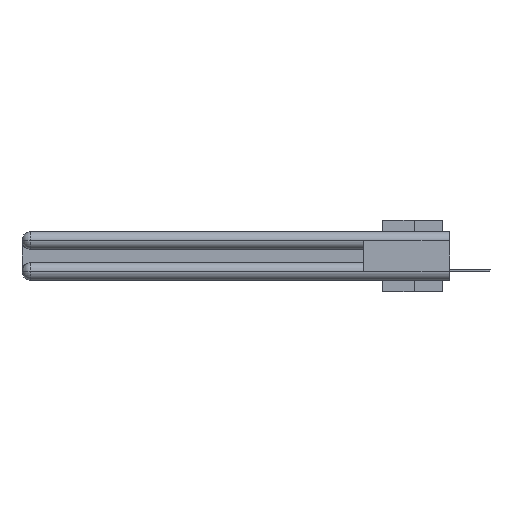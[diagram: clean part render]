
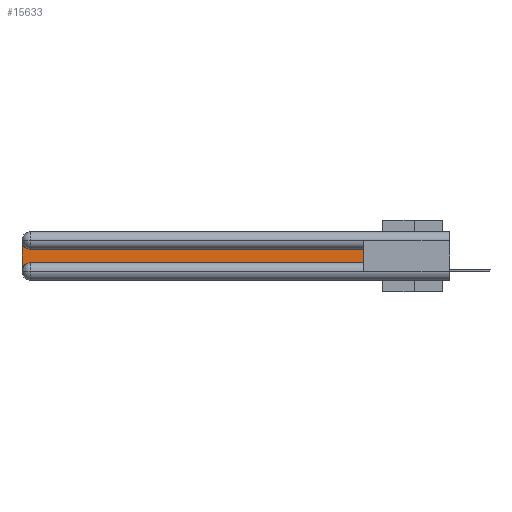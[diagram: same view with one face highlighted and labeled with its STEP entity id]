
A CAD part, left-side view. The second image highlights one B-rep face of the part: STEP entity #15633.
In plain terms, the highlighted planar face has unit normal (-1, 0, 0).
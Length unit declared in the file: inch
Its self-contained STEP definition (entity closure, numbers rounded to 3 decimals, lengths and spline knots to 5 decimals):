
#83 = DIRECTION ( 'NONE',  ( 1., 0., 0. ) ) ;
#89 = LINE ( 'NONE', #3940, #10854 ) ;
#229 = CARTESIAN_POINT ( 'NONE',  ( 0.075, 3., -0.1225 ) ) ;
#398 = LINE ( 'NONE', #16155, #8438 ) ;
#1423 = CARTESIAN_POINT ( 'NONE',  ( 0.075, 2.94, -0.2175 ) ) ;
#2996 = LINE ( 'NONE', #21391, #3380 ) ;
#3380 = VECTOR ( 'NONE', #16532, 39.37008 ) ;
#3928 = ORIENTED_EDGE ( 'NONE', *, *, #16909, .T. ) ;
#3940 = CARTESIAN_POINT ( 'NONE',  ( 0.075, 0.6, -0.1225 ) ) ;
#4543 = EDGE_CURVE ( 'NONE', #19600, #17707, #19312, .T. ) ;
#7042 = DIRECTION ( 'NONE',  ( 0., 0., -1. ) ) ;
#7452 = PLANE ( 'NONE',  #21684 ) ;
#7668 = DIRECTION ( 'NONE',  ( 0., 0., -1. ) ) ;
#7997 = VERTEX_POINT ( 'NONE', #13344 ) ;
#8438 = VECTOR ( 'NONE', #7042, 39.37008 ) ;
#9821 = EDGE_CURVE ( 'NONE', #17707, #26002, #16033, .T. ) ;
#10376 = AXIS2_PLACEMENT_3D ( 'NONE', #18546, #18969, #7668 ) ;
#10854 = VECTOR ( 'NONE', #15255, 39.37008 ) ;
#11321 = DIRECTION ( 'NONE',  ( 0., -1., 0. ) ) ;
#12529 = ORIENTED_EDGE ( 'NONE', *, *, #9821, .T. ) ;
#13344 = CARTESIAN_POINT ( 'NONE',  ( 0.075, 3., -0.0625 ) ) ;
#13564 = ORIENTED_EDGE ( 'NONE', *, *, #24252, .T. ) ;
#13764 = FACE_OUTER_BOUND ( 'NONE', #17303, .T. ) ;
#15255 = DIRECTION ( 'NONE',  ( 0., 1., 0. ) ) ;
#15517 = CARTESIAN_POINT ( 'NONE',  ( 0.075, 3., -0.2775 ) ) ;
#15633 = ADVANCED_FACE ( 'NONE', ( #13764 ), #7452, .F. ) ;
#15836 = VECTOR ( 'NONE', #11321, 39.37008 ) ;
#15968 = AXIS2_PLACEMENT_3D ( 'NONE', #19828, #20266, #24381 ) ;
#16033 = LINE ( 'NONE', #18380, #15836 ) ;
#16155 = CARTESIAN_POINT ( 'NONE',  ( 0.075, 3., -0.2175 ) ) ;
#16532 = DIRECTION ( 'NONE',  ( 0., 0., 1. ) ) ;
#16879 = CIRCLE ( 'NONE', #15968, 0.06 ) ;
#16909 = EDGE_CURVE ( 'NONE', #24529, #18511, #89, .T. ) ;
#17291 = ORIENTED_EDGE ( 'NONE', *, *, #4543, .T. ) ;
#17303 = EDGE_LOOP ( 'NONE', ( #3928, #13564, #19313, #17291, #12529, #22679 ) ) ;
#17707 = VERTEX_POINT ( 'NONE', #1423 ) ;
#17959 = EDGE_CURVE ( 'NONE', #26002, #24529, #2996, .T. ) ;
#18321 = DIRECTION ( 'NONE',  ( 0., 0., -1. ) ) ;
#18380 = CARTESIAN_POINT ( 'NONE',  ( 0.075, 0.6, -0.2175 ) ) ;
#18511 = VERTEX_POINT ( 'NONE', #28096 ) ;
#18546 = CARTESIAN_POINT ( 'NONE',  ( 0.075, 2.94, -0.2775 ) ) ;
#18969 = DIRECTION ( 'NONE',  ( 1., 0., 0. ) ) ;
#19312 = CIRCLE ( 'NONE', #10376, 0.06 ) ;
#19313 = ORIENTED_EDGE ( 'NONE', *, *, #24454, .T. ) ;
#19600 = VERTEX_POINT ( 'NONE', #15517 ) ;
#19828 = CARTESIAN_POINT ( 'NONE',  ( 0.075, 2.94, -0.0625 ) ) ;
#20266 = DIRECTION ( 'NONE',  ( 1., 0., 0. ) ) ;
#21391 = CARTESIAN_POINT ( 'NONE',  ( 0.075, 0.6, -0.2175 ) ) ;
#21684 = AXIS2_PLACEMENT_3D ( 'NONE', #229, #83, #18321 ) ;
#22679 = ORIENTED_EDGE ( 'NONE', *, *, #17959, .T. ) ;
#24252 = EDGE_CURVE ( 'NONE', #18511, #7997, #16879, .T. ) ;
#24381 = DIRECTION ( 'NONE',  ( 0., 0., -1. ) ) ;
#24454 = EDGE_CURVE ( 'NONE', #7997, #19600, #398, .T. ) ;
#24529 = VERTEX_POINT ( 'NONE', #25681 ) ;
#25681 = CARTESIAN_POINT ( 'NONE',  ( 0.075, 0.6, -0.1225 ) ) ;
#26002 = VERTEX_POINT ( 'NONE', #28149 ) ;
#28096 = CARTESIAN_POINT ( 'NONE',  ( 0.075, 2.94, -0.1225 ) ) ;
#28149 = CARTESIAN_POINT ( 'NONE',  ( 0.075, 0.6, -0.2175 ) ) ;
